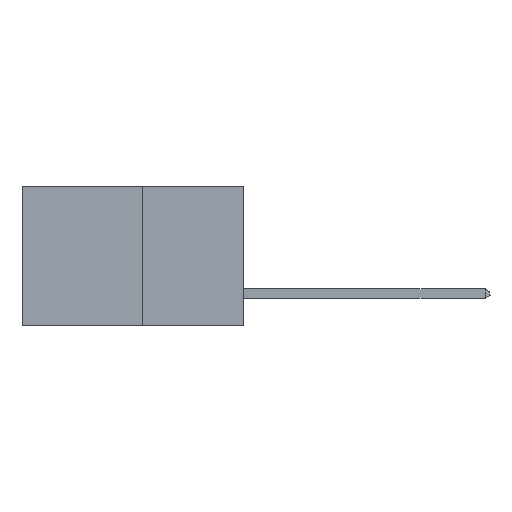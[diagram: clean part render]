
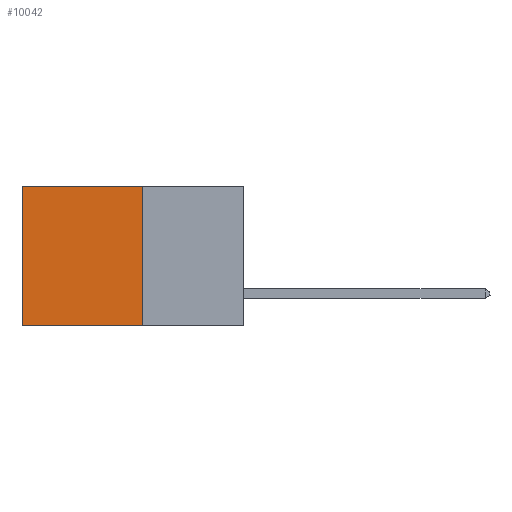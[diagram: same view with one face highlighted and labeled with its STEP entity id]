
A CAD part, left-side view. The second image highlights one B-rep face of the part: STEP entity #10042.
In plain terms, the highlighted planar face has unit normal (-1, 0, 0).
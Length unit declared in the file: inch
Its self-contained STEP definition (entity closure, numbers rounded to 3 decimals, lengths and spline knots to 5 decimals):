
#322 = ORIENTED_EDGE ( 'NONE', *, *, #12379, .F. ) ;
#611 = VECTOR ( 'NONE', #8856, 39.37008 ) ;
#717 = PLANE ( 'NONE',  #11862 ) ;
#944 = ORIENTED_EDGE ( 'NONE', *, *, #9772, .T. ) ;
#1205 = CARTESIAN_POINT ( 'NONE',  ( 0.277, 0.59, 0. ) ) ;
#1957 = CARTESIAN_POINT ( 'NONE',  ( 0.277, 0.27, -0.37 ) ) ;
#2075 = VERTEX_POINT ( 'NONE', #1957 ) ;
#2155 = VECTOR ( 'NONE', #4653, 39.37008 ) ;
#2428 = ORIENTED_EDGE ( 'NONE', *, *, #12324, .T. ) ;
#2441 = CARTESIAN_POINT ( 'NONE',  ( 0.277, 0.27, 0. ) ) ;
#2894 = ORIENTED_EDGE ( 'NONE', *, *, #6307, .F. ) ;
#3571 = CARTESIAN_POINT ( 'NONE',  ( 0.277, 0.59, -0.37 ) ) ;
#3656 = CARTESIAN_POINT ( 'NONE',  ( 0.277, 0.27, -0.37 ) ) ;
#3834 = LINE ( 'NONE', #2441, #611 ) ;
#3899 = CARTESIAN_POINT ( 'NONE',  ( 0.277, 0.59, -0.37 ) ) ;
#3944 = CARTESIAN_POINT ( 'NONE',  ( 0.277, 0.27, -0.37 ) ) ;
#4093 = EDGE_LOOP ( 'NONE', ( #2428, #2894, #322, #944 ) ) ;
#4444 = VECTOR ( 'NONE', #11033, 39.37008 ) ;
#4653 = DIRECTION ( 'NONE',  ( 0., 0., -1. ) ) ;
#5069 = DIRECTION ( 'NONE',  ( 0., 0., -1. ) ) ;
#6087 = CARTESIAN_POINT ( 'NONE',  ( 0.277, 0.27, 0. ) ) ;
#6307 = EDGE_CURVE ( 'NONE', #2075, #10004, #12427, .T. ) ;
#6830 = CARTESIAN_POINT ( 'NONE',  ( 0.277, 0.27, -0.37 ) ) ;
#8011 = FACE_OUTER_BOUND ( 'NONE', #4093, .T. ) ;
#8513 = VERTEX_POINT ( 'NONE', #1205 ) ;
#8856 = DIRECTION ( 'NONE',  ( 0., 1., 0. ) ) ;
#8981 = DIRECTION ( 'NONE',  ( 0., 0., -1. ) ) ;
#9772 = EDGE_CURVE ( 'NONE', #12546, #8513, #3834, .T. ) ;
#9994 = LINE ( 'NONE', #3656, #12349 ) ;
#10004 = VERTEX_POINT ( 'NONE', #3899 ) ;
#10042 = ADVANCED_FACE ( 'NONE', ( #8011 ), #717, .F. ) ;
#11033 = DIRECTION ( 'NONE',  ( 0., 1., 0. ) ) ;
#11372 = DIRECTION ( 'NONE',  ( 1., 0., 0. ) ) ;
#11862 = AXIS2_PLACEMENT_3D ( 'NONE', #3944, #11372, #5069 ) ;
#12324 = EDGE_CURVE ( 'NONE', #8513, #10004, #13258, .T. ) ;
#12349 = VECTOR ( 'NONE', #8981, 39.37008 ) ;
#12379 = EDGE_CURVE ( 'NONE', #12546, #2075, #9994, .T. ) ;
#12427 = LINE ( 'NONE', #6830, #4444 ) ;
#12546 = VERTEX_POINT ( 'NONE', #6087 ) ;
#13258 = LINE ( 'NONE', #3571, #2155 ) ;
